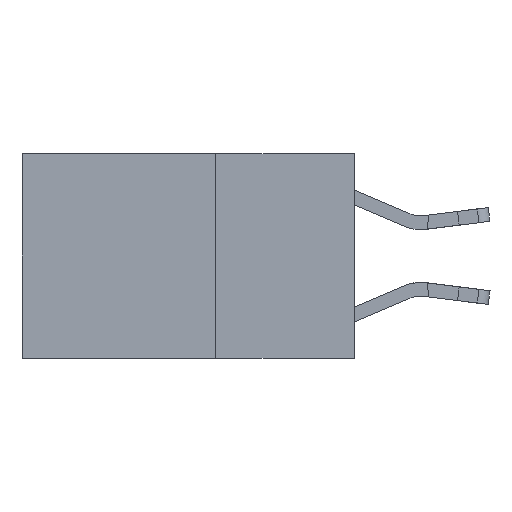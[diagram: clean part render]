
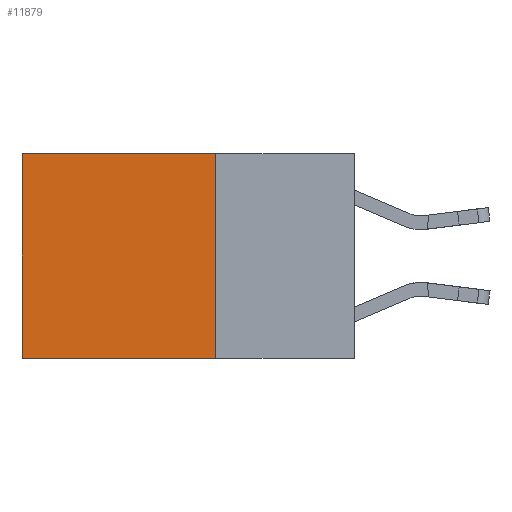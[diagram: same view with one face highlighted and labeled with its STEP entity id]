
A CAD part, left-side view. The second image highlights one B-rep face of the part: STEP entity #11879.
In plain terms, the highlighted planar face has unit normal (-1, 0, 0).
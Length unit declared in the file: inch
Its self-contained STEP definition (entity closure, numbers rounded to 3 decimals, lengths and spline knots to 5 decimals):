
#1273 = VECTOR ( 'NONE', #8205, 39.37008 ) ;
#2862 = CARTESIAN_POINT ( 'NONE',  ( 0.2625, 0.25, 0. ) ) ;
#3570 = CARTESIAN_POINT ( 'NONE',  ( 0.2625, 0.25, -0.37 ) ) ;
#4113 = ORIENTED_EDGE ( 'NONE', *, *, #7501, .T. ) ;
#4969 = VECTOR ( 'NONE', #21129, 39.37008 ) ;
#5037 = DIRECTION ( 'NONE',  ( 0., 0., -1. ) ) ;
#5960 = VERTEX_POINT ( 'NONE', #10541 ) ;
#6006 = CARTESIAN_POINT ( 'NONE',  ( 0.2625, 0.6, 0. ) ) ;
#6041 = CARTESIAN_POINT ( 'NONE',  ( 0.2625, 0.25, 0. ) ) ;
#6087 = EDGE_LOOP ( 'NONE', ( #4113, #16284, #23309, #16627 ) ) ;
#6947 = DIRECTION ( 'NONE',  ( 1., 0., 0. ) ) ;
#7162 = EDGE_CURVE ( 'NONE', #9404, #23976, #14852, .T. ) ;
#7185 = FACE_OUTER_BOUND ( 'NONE', #6087, .T. ) ;
#7501 = EDGE_CURVE ( 'NONE', #5960, #23976, #24194, .T. ) ;
#8205 = DIRECTION ( 'NONE',  ( 0., 0., -1. ) ) ;
#8314 = VERTEX_POINT ( 'NONE', #10766 ) ;
#8957 = AXIS2_PLACEMENT_3D ( 'NONE', #19852, #6947, #22006 ) ;
#9404 = VERTEX_POINT ( 'NONE', #3570 ) ;
#9811 = VECTOR ( 'NONE', #22143, 39.37008 ) ;
#10541 = CARTESIAN_POINT ( 'NONE',  ( 0.2625, 0.6, 0. ) ) ;
#10766 = CARTESIAN_POINT ( 'NONE',  ( 0.2625, 0.25, 0. ) ) ;
#11382 = LINE ( 'NONE', #2862, #27602 ) ;
#11879 = ADVANCED_FACE ( 'NONE', ( #7185 ), #15533, .F. ) ;
#13613 = CARTESIAN_POINT ( 'NONE',  ( 0.2625, 0.25, -0.37 ) ) ;
#14852 = LINE ( 'NONE', #13613, #9811 ) ;
#15533 = PLANE ( 'NONE',  #8957 ) ;
#15846 = EDGE_CURVE ( 'NONE', #8314, #5960, #20816, .T. ) ;
#16284 = ORIENTED_EDGE ( 'NONE', *, *, #7162, .F. ) ;
#16627 = ORIENTED_EDGE ( 'NONE', *, *, #15846, .T. ) ;
#19272 = EDGE_CURVE ( 'NONE', #8314, #9404, #11382, .T. ) ;
#19852 = CARTESIAN_POINT ( 'NONE',  ( 0.2625, 0.25, 0. ) ) ;
#20816 = LINE ( 'NONE', #6041, #4969 ) ;
#21129 = DIRECTION ( 'NONE',  ( 0., 1., 0. ) ) ;
#22006 = DIRECTION ( 'NONE',  ( 0., 0., -1. ) ) ;
#22143 = DIRECTION ( 'NONE',  ( 0., 1., 0. ) ) ;
#23309 = ORIENTED_EDGE ( 'NONE', *, *, #19272, .F. ) ;
#23976 = VERTEX_POINT ( 'NONE', #26227 ) ;
#24194 = LINE ( 'NONE', #6006, #1273 ) ;
#26227 = CARTESIAN_POINT ( 'NONE',  ( 0.2625, 0.6, -0.37 ) ) ;
#27602 = VECTOR ( 'NONE', #5037, 39.37008 ) ;
